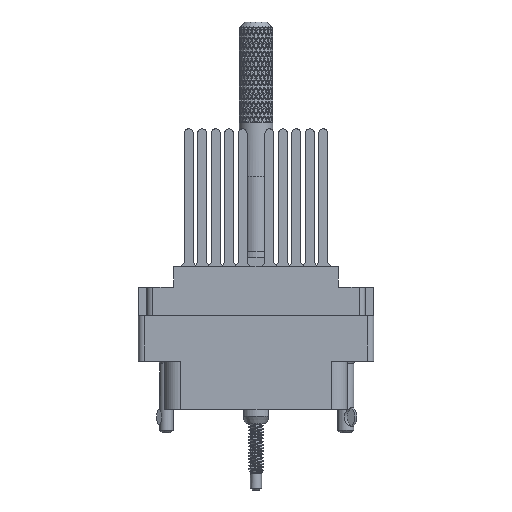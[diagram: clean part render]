
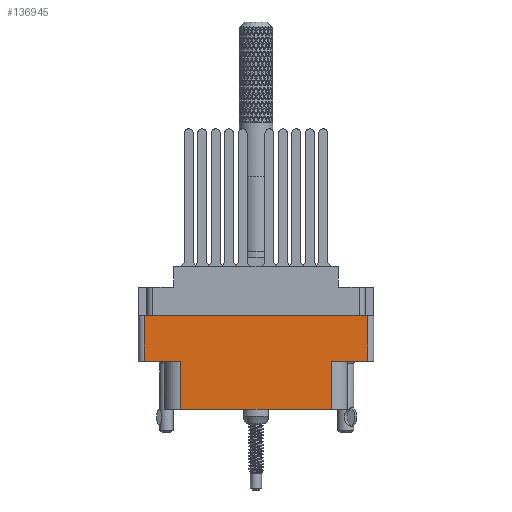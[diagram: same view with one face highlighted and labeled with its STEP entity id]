
A CAD part, front view. The second image highlights one B-rep face of the part: STEP entity #136945.
In plain terms, the highlighted planar face has unit normal (0, -1, 0).
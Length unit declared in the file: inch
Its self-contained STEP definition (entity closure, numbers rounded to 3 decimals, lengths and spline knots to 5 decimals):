
#1000 = VECTOR ( 'NONE', #87841, 39.37008 ) ;
#5444 = CARTESIAN_POINT ( 'NONE',  ( -0.42052, -0.343, -0.798 ) ) ;
#5757 = LINE ( 'NONE', #26690, #1000 ) ;
#6366 = VERTEX_POINT ( 'NONE', #53493 ) ;
#7353 = DIRECTION ( 'NONE',  ( 0., 0., -1. ) ) ;
#8021 = LINE ( 'NONE', #120143, #88887 ) ;
#11090 = CARTESIAN_POINT ( 'NONE',  ( 0.624, -0.343, -0.274 ) ) ;
#11470 = VECTOR ( 'NONE', #175474, 39.37008 ) ;
#15077 = DIRECTION ( 'NONE',  ( 1., 0., 0. ) ) ;
#15211 = CARTESIAN_POINT ( 'NONE',  ( 0.42052, -0.343, -0.529 ) ) ;
#23480 = ORIENTED_EDGE ( 'NONE', *, *, #190132, .T. ) ;
#26690 = CARTESIAN_POINT ( 'NONE',  ( 0., -0.343, -0.529 ) ) ;
#30448 = VERTEX_POINT ( 'NONE', #81114 ) ;
#33196 = PLANE ( 'NONE',  #42042 ) ;
#34787 = ORIENTED_EDGE ( 'NONE', *, *, #47544, .F. ) ;
#42042 = AXIS2_PLACEMENT_3D ( 'NONE', #141523, #78376, #50439 ) ;
#42605 = CARTESIAN_POINT ( 'NONE',  ( -0.624, -0.343, -0.274 ) ) ;
#43932 = ORIENTED_EDGE ( 'NONE', *, *, #147404, .T. ) ;
#45851 = VECTOR ( 'NONE', #166776, 39.37008 ) ;
#47544 = EDGE_CURVE ( 'NONE', #100392, #193309, #8021, .T. ) ;
#49077 = DIRECTION ( 'NONE',  ( 1., 0., 0. ) ) ;
#50439 = DIRECTION ( 'NONE',  ( 0., 0., -1. ) ) ;
#50625 = LINE ( 'NONE', #15211, #45851 ) ;
#53493 = CARTESIAN_POINT ( 'NONE',  ( 0.42052, -0.343, -0.798 ) ) ;
#54468 = CARTESIAN_POINT ( 'NONE',  ( -0.656, -0.343, -0.798 ) ) ;
#55889 = LINE ( 'NONE', #147032, #79771 ) ;
#57228 = VECTOR ( 'NONE', #49077, 39.37008 ) ;
#60030 = CARTESIAN_POINT ( 'NONE',  ( 0.624, -0.343, -0.798 ) ) ;
#72555 = CARTESIAN_POINT ( 'NONE',  ( -0.42052, -0.343, -0.798 ) ) ;
#77284 = VECTOR ( 'NONE', #90008, 39.37008 ) ;
#78376 = DIRECTION ( 'NONE',  ( 0., -1., 0. ) ) ;
#79771 = VECTOR ( 'NONE', #114545, 39.37008 ) ;
#81114 = CARTESIAN_POINT ( 'NONE',  ( -0.42052, -0.343, -0.529 ) ) ;
#81708 = EDGE_CURVE ( 'NONE', #93628, #196726, #5757, .T. ) ;
#85808 = VERTEX_POINT ( 'NONE', #108509 ) ;
#87841 = DIRECTION ( 'NONE',  ( -1., 0., 0. ) ) ;
#88733 = EDGE_CURVE ( 'NONE', #150066, #6366, #158937, .T. ) ;
#88887 = VECTOR ( 'NONE', #15077, 39.37008 ) ;
#90008 = DIRECTION ( 'NONE',  ( 0., 0., 1. ) ) ;
#93628 = VERTEX_POINT ( 'NONE', #98408 ) ;
#94372 = CARTESIAN_POINT ( 'NONE',  ( 0., -0.343, -0.529 ) ) ;
#94824 = LINE ( 'NONE', #5444, #116138 ) ;
#98408 = CARTESIAN_POINT ( 'NONE',  ( 0.624, -0.343, -0.529 ) ) ;
#100392 = VERTEX_POINT ( 'NONE', #42605 ) ;
#108509 = CARTESIAN_POINT ( 'NONE',  ( -0.624, -0.343, -0.529 ) ) ;
#114545 = DIRECTION ( 'NONE',  ( 0., 0., -1. ) ) ;
#116138 = VECTOR ( 'NONE', #7353, 39.37008 ) ;
#120143 = CARTESIAN_POINT ( 'NONE',  ( 0., -0.343, -0.274 ) ) ;
#128088 = EDGE_CURVE ( 'NONE', #30448, #150066, #94824, .T. ) ;
#136945 = ADVANCED_FACE ( 'NONE', ( #149049 ), #33196, .T. ) ;
#137761 = ORIENTED_EDGE ( 'NONE', *, *, #88733, .T. ) ;
#141523 = CARTESIAN_POINT ( 'NONE',  ( -0.656, -0.343, -0.798 ) ) ;
#147032 = CARTESIAN_POINT ( 'NONE',  ( -0.624, -0.343, -0.798 ) ) ;
#147404 = EDGE_CURVE ( 'NONE', #100392, #85808, #55889, .T. ) ;
#149049 = FACE_OUTER_BOUND ( 'NONE', #153950, .T. ) ;
#150066 = VERTEX_POINT ( 'NONE', #72555 ) ;
#153950 = EDGE_LOOP ( 'NONE', ( #34787, #43932, #23480, #174462, #137761, #169575, #170341, #161858 ) ) ;
#158937 = LINE ( 'NONE', #54468, #11470 ) ;
#161858 = ORIENTED_EDGE ( 'NONE', *, *, #183294, .T. ) ;
#166776 = DIRECTION ( 'NONE',  ( 0., 0., 1. ) ) ;
#169575 = ORIENTED_EDGE ( 'NONE', *, *, #187576, .T. ) ;
#170341 = ORIENTED_EDGE ( 'NONE', *, *, #81708, .F. ) ;
#173875 = LINE ( 'NONE', #94372, #57228 ) ;
#174462 = ORIENTED_EDGE ( 'NONE', *, *, #128088, .T. ) ;
#175474 = DIRECTION ( 'NONE',  ( 1., 0., 0. ) ) ;
#179723 = LINE ( 'NONE', #60030, #77284 ) ;
#183294 = EDGE_CURVE ( 'NONE', #93628, #193309, #179723, .T. ) ;
#187576 = EDGE_CURVE ( 'NONE', #6366, #196726, #50625, .T. ) ;
#190132 = EDGE_CURVE ( 'NONE', #85808, #30448, #173875, .T. ) ;
#193309 = VERTEX_POINT ( 'NONE', #11090 ) ;
#195517 = CARTESIAN_POINT ( 'NONE',  ( 0.42052, -0.343, -0.529 ) ) ;
#196726 = VERTEX_POINT ( 'NONE', #195517 ) ;
